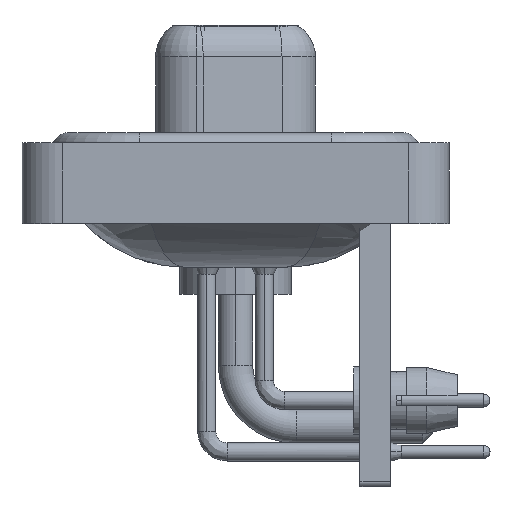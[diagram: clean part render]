
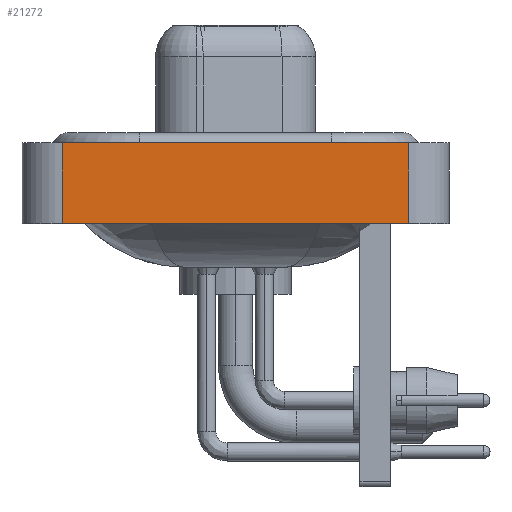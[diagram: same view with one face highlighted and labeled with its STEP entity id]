
A CAD part, left-side view. The second image highlights one B-rep face of the part: STEP entity #21272.
In plain terms, the highlighted planar face has unit normal (-1, 0, 0).
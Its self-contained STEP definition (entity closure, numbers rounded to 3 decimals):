
#453 = PLANE ( 'NONE',  #10664 ) ;
#1825 = CARTESIAN_POINT ( 'NONE',  ( -7.35, 8.55, -3.6 ) ) ;
#1938 = CARTESIAN_POINT ( 'NONE',  ( -7.35, 8.55, 0.4 ) ) ;
#2457 = LINE ( 'NONE', #13228, #11267 ) ;
#4480 = ORIENTED_EDGE ( 'NONE', *, *, #8110, .T. ) ;
#4955 = VECTOR ( 'NONE', #25327, 1000. ) ;
#5136 = EDGE_LOOP ( 'NONE', ( #21999, #9002, #15539, #4480 ) ) ;
#5217 = CARTESIAN_POINT ( 'NONE',  ( -7.35, -8.55, 0.4 ) ) ;
#5234 = EDGE_CURVE ( 'NONE', #24456, #6657, #2457, .T. ) ;
#6657 = VERTEX_POINT ( 'NONE', #26241 ) ;
#7064 = EDGE_CURVE ( 'NONE', #14495, #23028, #26631, .T. ) ;
#8110 = EDGE_CURVE ( 'NONE', #14495, #24456, #11603, .T. ) ;
#8580 = EDGE_CURVE ( 'NONE', #23028, #6657, #18853, .T. ) ;
#9002 = ORIENTED_EDGE ( 'NONE', *, *, #8580, .F. ) ;
#10664 = AXIS2_PLACEMENT_3D ( 'NONE', #22002, #15408, #13248 ) ;
#10727 = DIRECTION ( 'NONE',  ( 0., 0., 1. ) ) ;
#11267 = VECTOR ( 'NONE', #24310, 1000. ) ;
#11603 = LINE ( 'NONE', #14063, #4955 ) ;
#11890 = CARTESIAN_POINT ( 'NONE',  ( -7.35, -8.55, -3.6 ) ) ;
#13228 = CARTESIAN_POINT ( 'NONE',  ( -7.35, -8.55, -3.6 ) ) ;
#13248 = DIRECTION ( 'NONE',  ( 0., 0., 1. ) ) ;
#14063 = CARTESIAN_POINT ( 'NONE',  ( -7.35, -8.55, -3.6 ) ) ;
#14495 = VERTEX_POINT ( 'NONE', #24526 ) ;
#15408 = DIRECTION ( 'NONE',  ( -1., 0., 0. ) ) ;
#15539 = ORIENTED_EDGE ( 'NONE', *, *, #7064, .F. ) ;
#18853 = LINE ( 'NONE', #5217, #28228 ) ;
#20226 = FACE_OUTER_BOUND ( 'NONE', #5136, .T. ) ;
#21272 = ADVANCED_FACE ( 'NONE', ( #20226 ), #453, .T. ) ;
#21999 = ORIENTED_EDGE ( 'NONE', *, *, #5234, .T. ) ;
#22002 = CARTESIAN_POINT ( 'NONE',  ( -7.35, -8.55, -3.6 ) ) ;
#23028 = VERTEX_POINT ( 'NONE', #1938 ) ;
#24310 = DIRECTION ( 'NONE',  ( 0., 0., 1. ) ) ;
#24456 = VERTEX_POINT ( 'NONE', #11890 ) ;
#24526 = CARTESIAN_POINT ( 'NONE',  ( -7.35, 8.55, -3.6 ) ) ;
#24724 = VECTOR ( 'NONE', #10727, 1000. ) ;
#25327 = DIRECTION ( 'NONE',  ( 0., -1., 0. ) ) ;
#26241 = CARTESIAN_POINT ( 'NONE',  ( -7.35, -8.55, 0.4 ) ) ;
#26631 = LINE ( 'NONE', #1825, #24724 ) ;
#27514 = DIRECTION ( 'NONE',  ( 0., -1., 0. ) ) ;
#28228 = VECTOR ( 'NONE', #27514, 1000. ) ;
